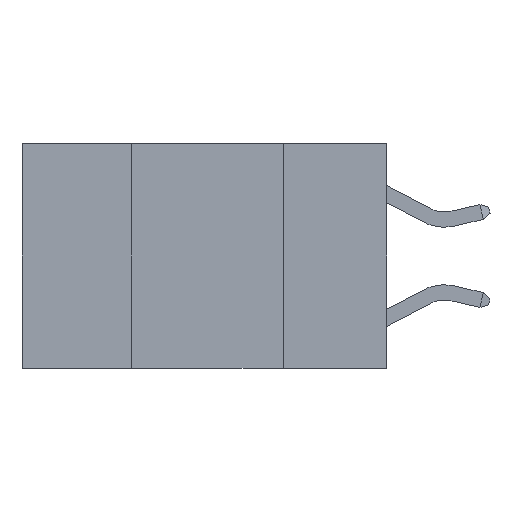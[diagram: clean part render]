
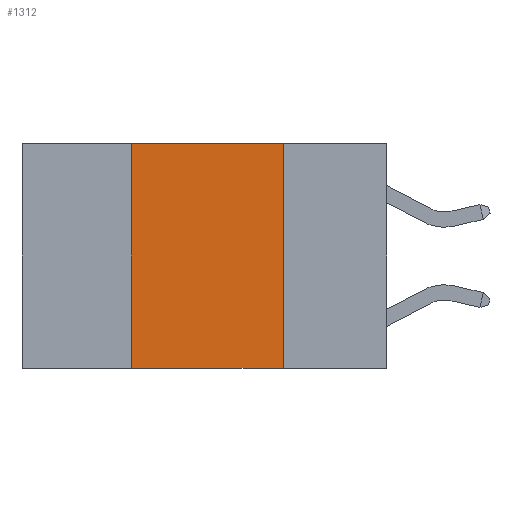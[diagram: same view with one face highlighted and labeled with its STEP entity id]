
A CAD part, left-side view. The second image highlights one B-rep face of the part: STEP entity #1312.
In plain terms, the highlighted planar face has unit normal (-1, 0, 0).
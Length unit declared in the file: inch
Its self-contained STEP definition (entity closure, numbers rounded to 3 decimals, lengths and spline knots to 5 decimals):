
#5 = EDGE_CURVE ( 'NONE', #10824, #2714, #9461, .T. ) ;
#1312 = ADVANCED_FACE ( 'NONE', ( #5113 ), #13241, .F. ) ;
#1744 = EDGE_LOOP ( 'NONE', ( #3614, #3868, #11908, #9545 ) ) ;
#2139 = DIRECTION ( 'NONE',  ( 0., 0., -1. ) ) ;
#2391 = VERTEX_POINT ( 'NONE', #15421 ) ;
#2714 = VERTEX_POINT ( 'NONE', #6260 ) ;
#2746 = EDGE_CURVE ( 'NONE', #10824, #13693, #3422, .T. ) ;
#3422 = LINE ( 'NONE', #7231, #6435 ) ;
#3614 = ORIENTED_EDGE ( 'NONE', *, *, #7057, .F. ) ;
#3868 = ORIENTED_EDGE ( 'NONE', *, *, #15140, .F. ) ;
#5113 = FACE_OUTER_BOUND ( 'NONE', #1744, .T. ) ;
#5483 = CARTESIAN_POINT ( 'NONE',  ( 0., 0.17, 0. ) ) ;
#5591 = VECTOR ( 'NONE', #14156, 39.37008 ) ;
#5712 = CARTESIAN_POINT ( 'NONE',  ( 0., 0.6, -0.37 ) ) ;
#6147 = VECTOR ( 'NONE', #7461, 39.37008 ) ;
#6260 = CARTESIAN_POINT ( 'NONE',  ( 0., 0.17, -0.37 ) ) ;
#6435 = VECTOR ( 'NONE', #11729, 39.37008 ) ;
#6458 = DIRECTION ( 'NONE',  ( 0., -1., 0. ) ) ;
#7057 = EDGE_CURVE ( 'NONE', #2391, #2714, #15427, .T. ) ;
#7231 = CARTESIAN_POINT ( 'NONE',  ( 0., 0.42, 0. ) ) ;
#7461 = DIRECTION ( 'NONE',  ( 0., -1., 0. ) ) ;
#9461 = LINE ( 'NONE', #5712, #6147 ) ;
#9545 = ORIENTED_EDGE ( 'NONE', *, *, #5, .T. ) ;
#10116 = CARTESIAN_POINT ( 'NONE',  ( 0., 0.6, 0. ) ) ;
#10289 = AXIS2_PLACEMENT_3D ( 'NONE', #13188, #10989, #2139 ) ;
#10824 = VERTEX_POINT ( 'NONE', #14141 ) ;
#10989 = DIRECTION ( 'NONE',  ( 1., 0., 0. ) ) ;
#11658 = LINE ( 'NONE', #10116, #14549 ) ;
#11729 = DIRECTION ( 'NONE',  ( 0., 0., 1. ) ) ;
#11908 = ORIENTED_EDGE ( 'NONE', *, *, #2746, .F. ) ;
#13188 = CARTESIAN_POINT ( 'NONE',  ( 0., 0.6, 0. ) ) ;
#13241 = PLANE ( 'NONE',  #10289 ) ;
#13660 = CARTESIAN_POINT ( 'NONE',  ( 0., 0.42, 0. ) ) ;
#13693 = VERTEX_POINT ( 'NONE', #13660 ) ;
#14141 = CARTESIAN_POINT ( 'NONE',  ( 0., 0.42, -0.37 ) ) ;
#14156 = DIRECTION ( 'NONE',  ( 0., 0., -1. ) ) ;
#14549 = VECTOR ( 'NONE', #6458, 39.37008 ) ;
#15140 = EDGE_CURVE ( 'NONE', #13693, #2391, #11658, .T. ) ;
#15421 = CARTESIAN_POINT ( 'NONE',  ( 0., 0.17, 0. ) ) ;
#15427 = LINE ( 'NONE', #5483, #5591 ) ;
